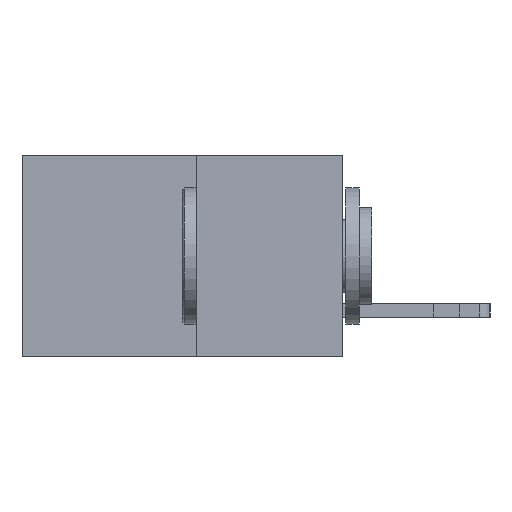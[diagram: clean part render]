
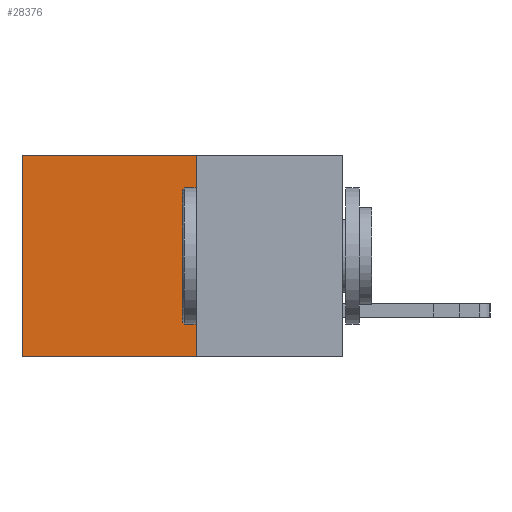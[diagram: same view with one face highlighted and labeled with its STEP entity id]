
A CAD part, left-side view. The second image highlights one B-rep face of the part: STEP entity #28376.
In plain terms, the highlighted planar face has unit normal (-1, 0, 0).
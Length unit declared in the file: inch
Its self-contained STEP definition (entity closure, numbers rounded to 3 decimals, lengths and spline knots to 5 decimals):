
#906 = ORIENTED_EDGE ( 'NONE', *, *, #29745, .T. ) ;
#1317 = CARTESIAN_POINT ( 'NONE',  ( 0.277, 0.59, -0.37 ) ) ;
#1551 = VECTOR ( 'NONE', #7247, 39.37008 ) ;
#2531 = VERTEX_POINT ( 'NONE', #28053 ) ;
#3639 = VECTOR ( 'NONE', #27618, 39.37008 ) ;
#4400 = LINE ( 'NONE', #22881, #3639 ) ;
#4929 = DIRECTION ( 'NONE',  ( 0., 1., 0. ) ) ;
#5112 = VERTEX_POINT ( 'NONE', #1317 ) ;
#6806 = PLANE ( 'NONE',  #29757 ) ;
#7247 = DIRECTION ( 'NONE',  ( 0., 1., 0. ) ) ;
#7598 = EDGE_CURVE ( 'NONE', #2531, #5112, #27818, .T. ) ;
#8186 = EDGE_LOOP ( 'NONE', ( #26749, #16407, #29707, #906 ) ) ;
#9989 = CARTESIAN_POINT ( 'NONE',  ( 0.277, 0.27, -0.37 ) ) ;
#11683 = DIRECTION ( 'NONE',  ( 0., 0., -1. ) ) ;
#12241 = VERTEX_POINT ( 'NONE', #9989 ) ;
#13250 = FACE_OUTER_BOUND ( 'NONE', #8186, .T. ) ;
#15015 = VECTOR ( 'NONE', #4929, 39.37008 ) ;
#16407 = ORIENTED_EDGE ( 'NONE', *, *, #21282, .F. ) ;
#16871 = DIRECTION ( 'NONE',  ( 0., 0., -1. ) ) ;
#17854 = EDGE_CURVE ( 'NONE', #21884, #12241, #4400, .T. ) ;
#19295 = CARTESIAN_POINT ( 'NONE',  ( 0.277, 0.27, 0. ) ) ;
#20739 = LINE ( 'NONE', #23961, #1551 ) ;
#20778 = VECTOR ( 'NONE', #16871, 39.37008 ) ;
#21282 = EDGE_CURVE ( 'NONE', #12241, #5112, #20739, .T. ) ;
#21325 = LINE ( 'NONE', #19295, #15015 ) ;
#21628 = CARTESIAN_POINT ( 'NONE',  ( 0.277, 0.59, -0.37 ) ) ;
#21884 = VERTEX_POINT ( 'NONE', #29651 ) ;
#22881 = CARTESIAN_POINT ( 'NONE',  ( 0.277, 0.27, -0.37 ) ) ;
#23532 = CARTESIAN_POINT ( 'NONE',  ( 0.277, 0.27, -0.37 ) ) ;
#23961 = CARTESIAN_POINT ( 'NONE',  ( 0.277, 0.27, -0.37 ) ) ;
#25919 = DIRECTION ( 'NONE',  ( 1., 0., 0. ) ) ;
#26749 = ORIENTED_EDGE ( 'NONE', *, *, #7598, .T. ) ;
#27618 = DIRECTION ( 'NONE',  ( 0., 0., -1. ) ) ;
#27818 = LINE ( 'NONE', #21628, #20778 ) ;
#28053 = CARTESIAN_POINT ( 'NONE',  ( 0.277, 0.59, 0. ) ) ;
#28376 = ADVANCED_FACE ( 'NONE', ( #13250 ), #6806, .F. ) ;
#29651 = CARTESIAN_POINT ( 'NONE',  ( 0.277, 0.27, 0. ) ) ;
#29707 = ORIENTED_EDGE ( 'NONE', *, *, #17854, .F. ) ;
#29745 = EDGE_CURVE ( 'NONE', #21884, #2531, #21325, .T. ) ;
#29757 = AXIS2_PLACEMENT_3D ( 'NONE', #23532, #25919, #11683 ) ;
